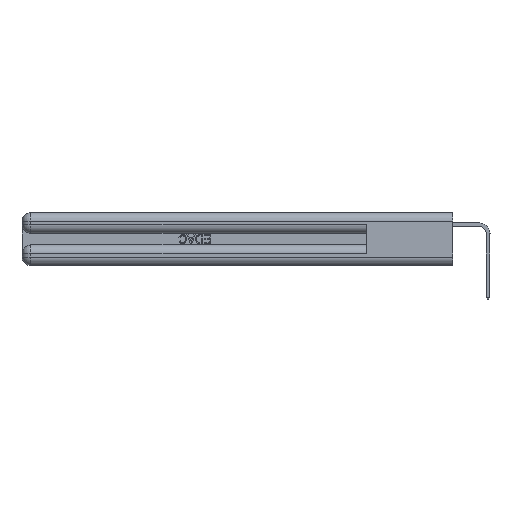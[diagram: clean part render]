
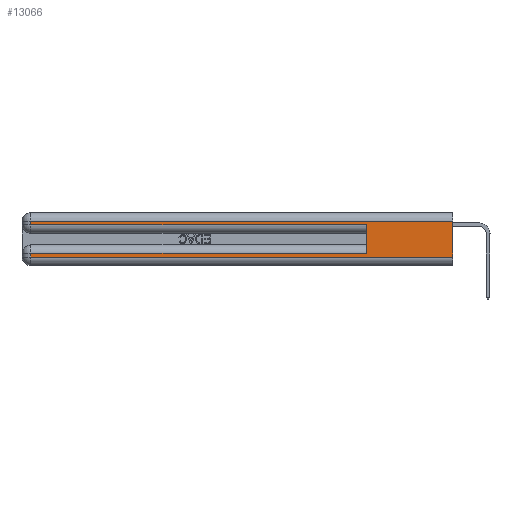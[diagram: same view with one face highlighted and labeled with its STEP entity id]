
A CAD part, left-side view. The second image highlights one B-rep face of the part: STEP entity #13066.
In plain terms, the highlighted planar face has unit normal (-1, 0, 0).
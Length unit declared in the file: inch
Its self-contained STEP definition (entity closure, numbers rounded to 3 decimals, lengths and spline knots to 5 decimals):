
#176 = CARTESIAN_POINT ( 'NONE',  ( 0., 0., 0.285 ) ) ;
#379 = EDGE_CURVE ( 'NONE', #15390, #7352, #34244, .T. ) ;
#836 = PLANE ( 'NONE',  #12052 ) ;
#1136 = LINE ( 'NONE', #30836, #27814 ) ;
#1152 = LINE ( 'NONE', #176, #19308 ) ;
#1856 = CARTESIAN_POINT ( 'NONE',  ( 0., 2.94, 0.085 ) ) ;
#3114 = VECTOR ( 'NONE', #28985, 39.37008 ) ;
#3261 = CARTESIAN_POINT ( 'NONE',  ( 0., 0.6, 0.145 ) ) ;
#3472 = ORIENTED_EDGE ( 'NONE', *, *, #30549, .F. ) ;
#3932 = EDGE_CURVE ( 'NONE', #21207, #7790, #5361, .T. ) ;
#3978 = ORIENTED_EDGE ( 'NONE', *, *, #14791, .T. ) ;
#4855 = CARTESIAN_POINT ( 'NONE',  ( 0., 0., 0.06 ) ) ;
#5243 = VERTEX_POINT ( 'NONE', #19883 ) ;
#5361 = LINE ( 'NONE', #11513, #29992 ) ;
#6737 = DIRECTION ( 'NONE',  ( 0., -1., 0. ) ) ;
#6946 = EDGE_CURVE ( 'NONE', #6948, #15390, #8216, .T. ) ;
#6948 = VERTEX_POINT ( 'NONE', #1856 ) ;
#7193 = VECTOR ( 'NONE', #33966, 39.37008 ) ;
#7206 = VERTEX_POINT ( 'NONE', #25753 ) ;
#7352 = VERTEX_POINT ( 'NONE', #10799 ) ;
#7790 = VERTEX_POINT ( 'NONE', #19225 ) ;
#8216 = LINE ( 'NONE', #24374, #7193 ) ;
#8236 = CARTESIAN_POINT ( 'NONE',  ( 0., 0., 0.085 ) ) ;
#8474 = DIRECTION ( 'NONE',  ( 0., 0., -1. ) ) ;
#10799 = CARTESIAN_POINT ( 'NONE',  ( 0., 0., 0.06 ) ) ;
#11513 = CARTESIAN_POINT ( 'NONE',  ( 0., 2.94, 0.37 ) ) ;
#11790 = LINE ( 'NONE', #3261, #3114 ) ;
#12052 = AXIS2_PLACEMENT_3D ( 'NONE', #23228, #36146, #17072 ) ;
#13066 = ADVANCED_FACE ( 'NONE', ( #31124 ), #836, .F. ) ;
#13908 = CARTESIAN_POINT ( 'NONE',  ( 0., 2.94, 0.06 ) ) ;
#14791 = EDGE_CURVE ( 'NONE', #14927, #21207, #33942, .T. ) ;
#14927 = VERTEX_POINT ( 'NONE', #21334 ) ;
#15390 = VERTEX_POINT ( 'NONE', #13908 ) ;
#15590 = EDGE_CURVE ( 'NONE', #7206, #6948, #31405, .T. ) ;
#17072 = DIRECTION ( 'NONE',  ( 0., 0., -1. ) ) ;
#17139 = ORIENTED_EDGE ( 'NONE', *, *, #379, .T. ) ;
#19112 = EDGE_LOOP ( 'NONE', ( #26622, #3978, #23125, #34570, #3472, #22633, #33116, #17139 ) ) ;
#19225 = CARTESIAN_POINT ( 'NONE',  ( 0., 2.94, 0.285 ) ) ;
#19308 = VECTOR ( 'NONE', #6737, 39.37008 ) ;
#19883 = CARTESIAN_POINT ( 'NONE',  ( 0., 0.6, 0.285 ) ) ;
#21207 = VERTEX_POINT ( 'NONE', #25234 ) ;
#21334 = CARTESIAN_POINT ( 'NONE',  ( 0., 0., 0.31 ) ) ;
#22633 = ORIENTED_EDGE ( 'NONE', *, *, #15590, .T. ) ;
#23125 = ORIENTED_EDGE ( 'NONE', *, *, #3932, .T. ) ;
#23228 = CARTESIAN_POINT ( 'NONE',  ( 0., 0., 0.37 ) ) ;
#24204 = DIRECTION ( 'NONE',  ( 0., 0., -1. ) ) ;
#24208 = DIRECTION ( 'NONE',  ( 0., 1., 0. ) ) ;
#24374 = CARTESIAN_POINT ( 'NONE',  ( 0., 2.94, 0.37 ) ) ;
#25234 = CARTESIAN_POINT ( 'NONE',  ( 0., 2.94, 0.31 ) ) ;
#25753 = CARTESIAN_POINT ( 'NONE',  ( 0., 0.6, 0.085 ) ) ;
#26511 = VECTOR ( 'NONE', #36613, 39.37008 ) ;
#26622 = ORIENTED_EDGE ( 'NONE', *, *, #27641, .F. ) ;
#27350 = DIRECTION ( 'NONE',  ( 0., -1., 0. ) ) ;
#27641 = EDGE_CURVE ( 'NONE', #14927, #7352, #1136, .T. ) ;
#27814 = VECTOR ( 'NONE', #8474, 39.37008 ) ;
#28985 = DIRECTION ( 'NONE',  ( 0., 0., 1. ) ) ;
#29992 = VECTOR ( 'NONE', #24204, 39.37008 ) ;
#30407 = VECTOR ( 'NONE', #24208, 39.37008 ) ;
#30549 = EDGE_CURVE ( 'NONE', #7206, #5243, #11790, .T. ) ;
#30836 = CARTESIAN_POINT ( 'NONE',  ( 0., 0., 0.37 ) ) ;
#31124 = FACE_OUTER_BOUND ( 'NONE', #19112, .T. ) ;
#31405 = LINE ( 'NONE', #8236, #30407 ) ;
#33116 = ORIENTED_EDGE ( 'NONE', *, *, #6946, .T. ) ;
#33453 = CARTESIAN_POINT ( 'NONE',  ( 0., 0., 0.31 ) ) ;
#33942 = LINE ( 'NONE', #33453, #26511 ) ;
#33966 = DIRECTION ( 'NONE',  ( 0., 0., -1. ) ) ;
#34244 = LINE ( 'NONE', #4855, #36231 ) ;
#34570 = ORIENTED_EDGE ( 'NONE', *, *, #39014, .T. ) ;
#36146 = DIRECTION ( 'NONE',  ( 1., 0., 0. ) ) ;
#36231 = VECTOR ( 'NONE', #27350, 39.37008 ) ;
#36613 = DIRECTION ( 'NONE',  ( 0., 1., 0. ) ) ;
#39014 = EDGE_CURVE ( 'NONE', #7790, #5243, #1152, .T. ) ;
